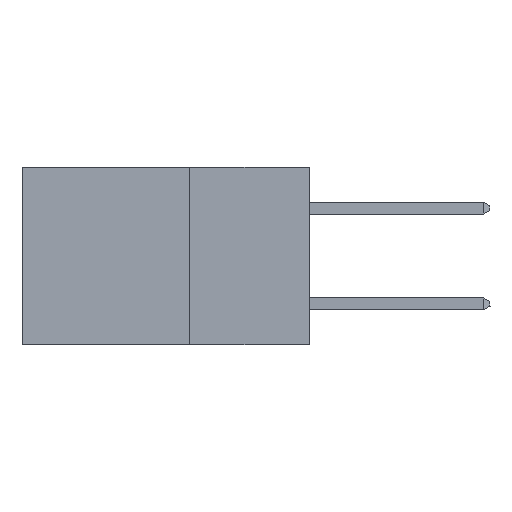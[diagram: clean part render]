
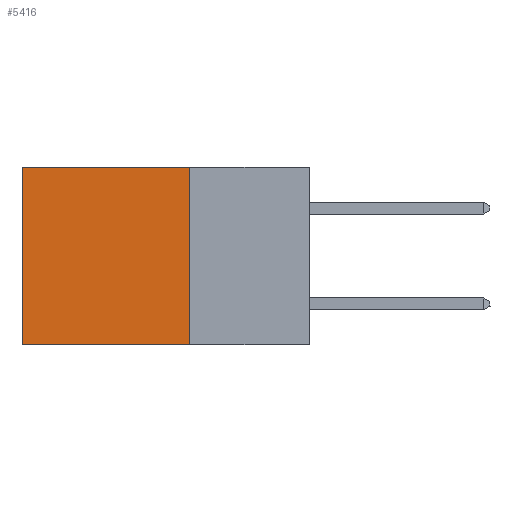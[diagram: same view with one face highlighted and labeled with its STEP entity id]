
A CAD part, left-side view. The second image highlights one B-rep face of the part: STEP entity #5416.
In plain terms, the highlighted planar face has unit normal (-1, 0, 0).
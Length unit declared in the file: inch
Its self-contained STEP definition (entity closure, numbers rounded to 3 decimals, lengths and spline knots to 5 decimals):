
#99 = CARTESIAN_POINT ( 'NONE',  ( 0.2875, 0.25, 0. ) ) ;
#117 = VERTEX_POINT ( 'NONE', #6044 ) ;
#220 = VECTOR ( 'NONE', #9492, 39.37008 ) ;
#566 = ORIENTED_EDGE ( 'NONE', *, *, #11167, .F. ) ;
#957 = CARTESIAN_POINT ( 'NONE',  ( 0.2875, 0.6, 0. ) ) ;
#1800 = VERTEX_POINT ( 'NONE', #2287 ) ;
#2037 = PLANE ( 'NONE',  #11507 ) ;
#2287 = CARTESIAN_POINT ( 'NONE',  ( 0.2875, 0.25, -0.37 ) ) ;
#2404 = CARTESIAN_POINT ( 'NONE',  ( 0.2875, 0.25, 0. ) ) ;
#3143 = DIRECTION ( 'NONE',  ( 0., 0., -1. ) ) ;
#3789 = LINE ( 'NONE', #6433, #6478 ) ;
#3798 = CARTESIAN_POINT ( 'NONE',  ( 0.2875, 0.25, -0.37 ) ) ;
#4719 = VERTEX_POINT ( 'NONE', #957 ) ;
#4911 = EDGE_CURVE ( 'NONE', #10226, #1800, #12935, .T. ) ;
#5416 = ADVANCED_FACE ( 'NONE', ( #9033 ), #2037, .F. ) ;
#5623 = ORIENTED_EDGE ( 'NONE', *, *, #10780, .T. ) ;
#6044 = CARTESIAN_POINT ( 'NONE',  ( 0.2875, 0.6, -0.37 ) ) ;
#6433 = CARTESIAN_POINT ( 'NONE',  ( 0.2875, 0.6, 0. ) ) ;
#6478 = VECTOR ( 'NONE', #11016, 39.37008 ) ;
#6499 = LINE ( 'NONE', #8239, #8838 ) ;
#7883 = DIRECTION ( 'NONE',  ( 0., 1., 0. ) ) ;
#8239 = CARTESIAN_POINT ( 'NONE',  ( 0.2875, 0.25, 0. ) ) ;
#8838 = VECTOR ( 'NONE', #12168, 39.37008 ) ;
#8937 = EDGE_LOOP ( 'NONE', ( #11722, #566, #11492, #5623 ) ) ;
#9033 = FACE_OUTER_BOUND ( 'NONE', #8937, .T. ) ;
#9166 = DIRECTION ( 'NONE',  ( 1., 0., 0. ) ) ;
#9492 = DIRECTION ( 'NONE',  ( 0., 0., -1. ) ) ;
#10033 = LINE ( 'NONE', #3798, #12383 ) ;
#10226 = VERTEX_POINT ( 'NONE', #99 ) ;
#10780 = EDGE_CURVE ( 'NONE', #10226, #4719, #6499, .T. ) ;
#11016 = DIRECTION ( 'NONE',  ( 0., 0., -1. ) ) ;
#11167 = EDGE_CURVE ( 'NONE', #1800, #117, #10033, .T. ) ;
#11492 = ORIENTED_EDGE ( 'NONE', *, *, #4911, .F. ) ;
#11507 = AXIS2_PLACEMENT_3D ( 'NONE', #13139, #9166, #3143 ) ;
#11673 = EDGE_CURVE ( 'NONE', #4719, #117, #3789, .T. ) ;
#11722 = ORIENTED_EDGE ( 'NONE', *, *, #11673, .T. ) ;
#12168 = DIRECTION ( 'NONE',  ( 0., 1., 0. ) ) ;
#12383 = VECTOR ( 'NONE', #7883, 39.37008 ) ;
#12935 = LINE ( 'NONE', #2404, #220 ) ;
#13139 = CARTESIAN_POINT ( 'NONE',  ( 0.2875, 0.25, 0. ) ) ;
